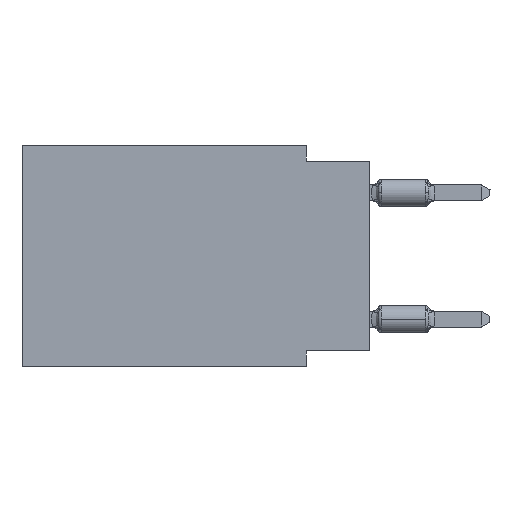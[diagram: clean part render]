
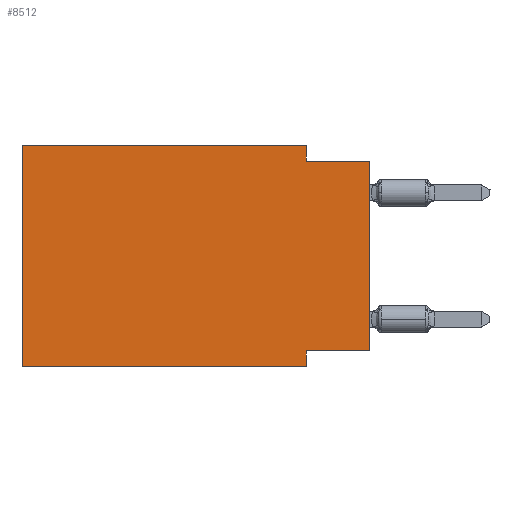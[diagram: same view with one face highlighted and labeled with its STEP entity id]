
A CAD part, left-side view. The second image highlights one B-rep face of the part: STEP entity #8512.
In plain terms, the highlighted planar face has unit normal (-1, 0, 0).
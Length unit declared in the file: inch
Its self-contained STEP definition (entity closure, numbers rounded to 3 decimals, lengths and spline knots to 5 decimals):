
#13 = DIRECTION ( 'NONE',  ( 0., 0., 1. ) ) ;
#201 = CARTESIAN_POINT ( 'NONE',  ( 0., 0.55, 0. ) ) ;
#797 = LINE ( 'NONE', #14397, #5567 ) ;
#1482 = CARTESIAN_POINT ( 'NONE',  ( 0., 0.55, 0. ) ) ;
#1804 = EDGE_CURVE ( 'NONE', #15410, #21505, #6341, .T. ) ;
#1868 = VECTOR ( 'NONE', #5773, 39.37008 ) ;
#1900 = ORIENTED_EDGE ( 'NONE', *, *, #6611, .F. ) ;
#2100 = CARTESIAN_POINT ( 'NONE',  ( 0., 0.55, -0.35 ) ) ;
#2152 = VECTOR ( 'NONE', #16068, 39.37008 ) ;
#2767 = CARTESIAN_POINT ( 'NONE',  ( 0., 0.55, 0. ) ) ;
#4449 = ORIENTED_EDGE ( 'NONE', *, *, #12657, .F. ) ;
#4869 = CARTESIAN_POINT ( 'NONE',  ( 0., 0., -0.325 ) ) ;
#5020 = FACE_OUTER_BOUND ( 'NONE', #22529, .T. ) ;
#5431 = ORIENTED_EDGE ( 'NONE', *, *, #8868, .T. ) ;
#5567 = VECTOR ( 'NONE', #7486, 39.37008 ) ;
#5773 = DIRECTION ( 'NONE',  ( 0., 0., -1. ) ) ;
#5906 = CARTESIAN_POINT ( 'NONE',  ( 0., 0.1, -0.35 ) ) ;
#6254 = EDGE_CURVE ( 'NONE', #12488, #9948, #20650, .T. ) ;
#6341 = LINE ( 'NONE', #2767, #14493 ) ;
#6611 = EDGE_CURVE ( 'NONE', #9948, #13437, #8088, .T. ) ;
#6963 = VECTOR ( 'NONE', #18334, 39.37008 ) ;
#7011 = DIRECTION ( 'NONE',  ( 1., 0., 0. ) ) ;
#7117 = ORIENTED_EDGE ( 'NONE', *, *, #11528, .F. ) ;
#7486 = DIRECTION ( 'NONE',  ( 0., 0., -1. ) ) ;
#8088 = LINE ( 'NONE', #5906, #1868 ) ;
#8130 = EDGE_CURVE ( 'NONE', #12488, #13204, #12430, .T. ) ;
#8246 = CARTESIAN_POINT ( 'NONE',  ( 0., 0.55, -0.35 ) ) ;
#8512 = ADVANCED_FACE ( 'NONE', ( #5020 ), #15975, .F. ) ;
#8868 = EDGE_CURVE ( 'NONE', #15410, #13437, #10072, .T. ) ;
#9055 = LINE ( 'NONE', #201, #2152 ) ;
#9172 = VECTOR ( 'NONE', #13, 39.37008 ) ;
#9948 = VERTEX_POINT ( 'NONE', #16545 ) ;
#10072 = LINE ( 'NONE', #8246, #17687 ) ;
#11040 = CARTESIAN_POINT ( 'NONE',  ( 0., 0.1, -0.35 ) ) ;
#11302 = VERTEX_POINT ( 'NONE', #21126 ) ;
#11528 = EDGE_CURVE ( 'NONE', #11302, #13204, #14886, .T. ) ;
#12054 = DIRECTION ( 'NONE',  ( 0., 0., -1. ) ) ;
#12156 = ORIENTED_EDGE ( 'NONE', *, *, #6254, .F. ) ;
#12324 = CARTESIAN_POINT ( 'NONE',  ( 0., 0., 0. ) ) ;
#12430 = LINE ( 'NONE', #12324, #9172 ) ;
#12488 = VERTEX_POINT ( 'NONE', #21841 ) ;
#12657 = EDGE_CURVE ( 'NONE', #21505, #15693, #9055, .T. ) ;
#13204 = VERTEX_POINT ( 'NONE', #22099 ) ;
#13437 = VERTEX_POINT ( 'NONE', #11040 ) ;
#14397 = CARTESIAN_POINT ( 'NONE',  ( 0., 0.1, 0. ) ) ;
#14493 = VECTOR ( 'NONE', #22443, 39.37008 ) ;
#14886 = LINE ( 'NONE', #16488, #6963 ) ;
#14934 = CARTESIAN_POINT ( 'NONE',  ( 0., 0.55, 0. ) ) ;
#15410 = VERTEX_POINT ( 'NONE', #2100 ) ;
#15693 = VERTEX_POINT ( 'NONE', #19552 ) ;
#15755 = ORIENTED_EDGE ( 'NONE', *, *, #8130, .T. ) ;
#15975 = PLANE ( 'NONE',  #19114 ) ;
#16068 = DIRECTION ( 'NONE',  ( 0., -1., 0. ) ) ;
#16419 = ORIENTED_EDGE ( 'NONE', *, *, #19610, .F. ) ;
#16488 = CARTESIAN_POINT ( 'NONE',  ( 0., 0., -0.025 ) ) ;
#16545 = CARTESIAN_POINT ( 'NONE',  ( 0., 0.1, -0.325 ) ) ;
#17687 = VECTOR ( 'NONE', #21825, 39.37008 ) ;
#17910 = ORIENTED_EDGE ( 'NONE', *, *, #1804, .F. ) ;
#18334 = DIRECTION ( 'NONE',  ( 0., -1., 0. ) ) ;
#19034 = DIRECTION ( 'NONE',  ( 0., 1., 0. ) ) ;
#19114 = AXIS2_PLACEMENT_3D ( 'NONE', #1482, #7011, #12054 ) ;
#19552 = CARTESIAN_POINT ( 'NONE',  ( 0., 0.1, 0. ) ) ;
#19610 = EDGE_CURVE ( 'NONE', #15693, #11302, #797, .T. ) ;
#19852 = VECTOR ( 'NONE', #19034, 39.37008 ) ;
#20650 = LINE ( 'NONE', #4869, #19852 ) ;
#21126 = CARTESIAN_POINT ( 'NONE',  ( 0., 0.1, -0.025 ) ) ;
#21505 = VERTEX_POINT ( 'NONE', #14934 ) ;
#21825 = DIRECTION ( 'NONE',  ( 0., -1., 0. ) ) ;
#21841 = CARTESIAN_POINT ( 'NONE',  ( 0., 0., -0.325 ) ) ;
#22099 = CARTESIAN_POINT ( 'NONE',  ( 0., 0., -0.025 ) ) ;
#22443 = DIRECTION ( 'NONE',  ( 0., 0., 1. ) ) ;
#22529 = EDGE_LOOP ( 'NONE', ( #15755, #7117, #16419, #4449, #17910, #5431, #1900, #12156 ) ) ;
